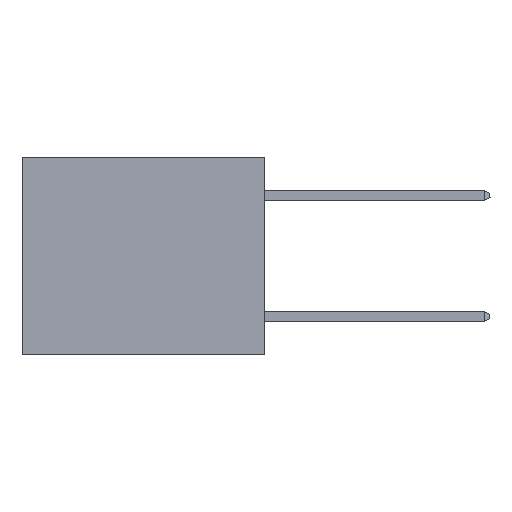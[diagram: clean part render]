
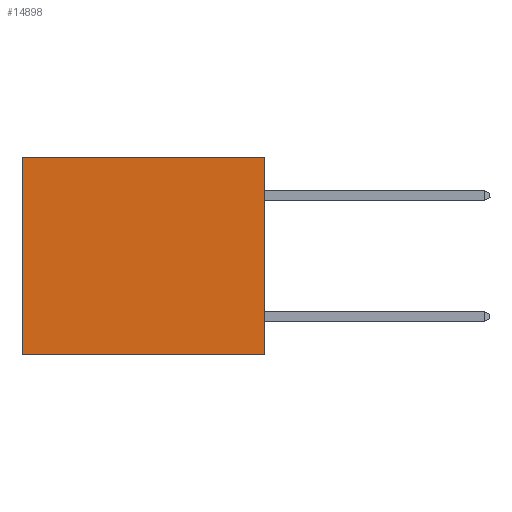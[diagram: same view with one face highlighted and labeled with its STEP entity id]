
A CAD part, left-side view. The second image highlights one B-rep face of the part: STEP entity #14898.
In plain terms, the highlighted planar face has unit normal (-1, 0, 0).
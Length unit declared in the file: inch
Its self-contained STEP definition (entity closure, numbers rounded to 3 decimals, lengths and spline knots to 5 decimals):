
#842 = AXIS2_PLACEMENT_3D ( 'NONE', #12490, #27968, #25750 ) ;
#1505 = LINE ( 'NONE', #17164, #24503 ) ;
#1506 = CARTESIAN_POINT ( 'NONE',  ( 0.3165, 0., 0. ) ) ;
#3092 = FACE_OUTER_BOUND ( 'NONE', #16209, .T. ) ;
#3537 = EDGE_CURVE ( 'NONE', #12616, #18210, #13510, .T. ) ;
#5318 = ORIENTED_EDGE ( 'NONE', *, *, #7142, .F. ) ;
#5351 = CARTESIAN_POINT ( 'NONE',  ( 0.3165, 0.6, -0.49 ) ) ;
#5778 = CARTESIAN_POINT ( 'NONE',  ( 0.3165, 0., -0.49 ) ) ;
#7142 = EDGE_CURVE ( 'NONE', #18120, #18210, #9862, .T. ) ;
#7987 = DIRECTION ( 'NONE',  ( 0., 0., -1. ) ) ;
#8805 = VECTOR ( 'NONE', #25511, 39.37008 ) ;
#9862 = LINE ( 'NONE', #9918, #8805 ) ;
#9918 = CARTESIAN_POINT ( 'NONE',  ( 0.3165, 0., -0.49 ) ) ;
#12490 = CARTESIAN_POINT ( 'NONE',  ( 0.3165, 0., -0.49 ) ) ;
#12616 = VERTEX_POINT ( 'NONE', #17224 ) ;
#13510 = LINE ( 'NONE', #5351, #24314 ) ;
#13860 = VERTEX_POINT ( 'NONE', #1506 ) ;
#14898 = ADVANCED_FACE ( 'NONE', ( #3092 ), #19191, .F. ) ;
#15951 = CARTESIAN_POINT ( 'NONE',  ( 0.3165, 0.6, -0.49 ) ) ;
#16209 = EDGE_LOOP ( 'NONE', ( #27241, #5318, #21798, #24884 ) ) ;
#16792 = EDGE_CURVE ( 'NONE', #13860, #12616, #1505, .T. ) ;
#17164 = CARTESIAN_POINT ( 'NONE',  ( 0.3165, 0., 0. ) ) ;
#17224 = CARTESIAN_POINT ( 'NONE',  ( 0.3165, 0.6, 0. ) ) ;
#18120 = VERTEX_POINT ( 'NONE', #18372 ) ;
#18210 = VERTEX_POINT ( 'NONE', #15951 ) ;
#18372 = CARTESIAN_POINT ( 'NONE',  ( 0.3165, 0., -0.49 ) ) ;
#19191 = PLANE ( 'NONE',  #842 ) ;
#21180 = VECTOR ( 'NONE', #7987, 39.37008 ) ;
#21537 = LINE ( 'NONE', #5778, #21180 ) ;
#21798 = ORIENTED_EDGE ( 'NONE', *, *, #24072, .F. ) ;
#23321 = DIRECTION ( 'NONE',  ( 0., 0., -1. ) ) ;
#24072 = EDGE_CURVE ( 'NONE', #13860, #18120, #21537, .T. ) ;
#24314 = VECTOR ( 'NONE', #23321, 39.37008 ) ;
#24503 = VECTOR ( 'NONE', #26033, 39.37008 ) ;
#24884 = ORIENTED_EDGE ( 'NONE', *, *, #16792, .T. ) ;
#25511 = DIRECTION ( 'NONE',  ( 0., 1., 0. ) ) ;
#25750 = DIRECTION ( 'NONE',  ( 0., 0., -1. ) ) ;
#26033 = DIRECTION ( 'NONE',  ( 0., 1., 0. ) ) ;
#27241 = ORIENTED_EDGE ( 'NONE', *, *, #3537, .T. ) ;
#27968 = DIRECTION ( 'NONE',  ( 1., 0., 0. ) ) ;
